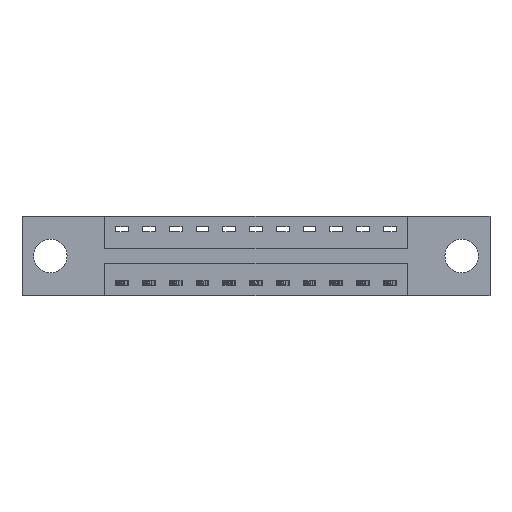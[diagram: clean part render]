
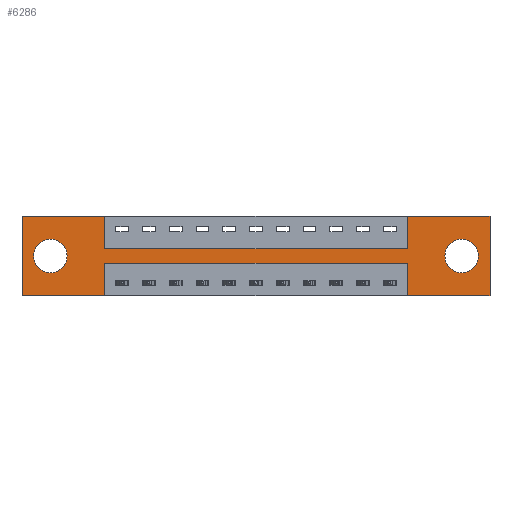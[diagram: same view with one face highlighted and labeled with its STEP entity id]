
A CAD part, front view. The second image highlights one B-rep face of the part: STEP entity #6286.
In plain terms, the highlighted planar face has unit normal (0, -1, 0).
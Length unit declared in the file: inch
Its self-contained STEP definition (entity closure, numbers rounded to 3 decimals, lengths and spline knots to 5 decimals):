
#177 = VERTEX_POINT ( 'NONE', #10046 ) ;
#226 = LINE ( 'NONE', #3728, #1477 ) ;
#584 = CARTESIAN_POINT ( 'NONE',  ( 2.0525, 0., -0.107 ) ) ;
#644 = DIRECTION ( 'NONE',  ( 1., 0., 0. ) ) ;
#660 = ORIENTED_EDGE ( 'NONE', *, *, #10519, .F. ) ;
#899 = DIRECTION ( 'NONE',  ( 0., 0., -1. ) ) ;
#930 = AXIS2_PLACEMENT_3D ( 'NONE', #1016, #8815, #899 ) ;
#969 = VERTEX_POINT ( 'NONE', #1313 ) ;
#1016 = CARTESIAN_POINT ( 'NONE',  ( 0., 0., -0.37 ) ) ;
#1032 = VERTEX_POINT ( 'NONE', #584 ) ;
#1133 = CARTESIAN_POINT ( 'NONE',  ( 0.3875, 0., -0.37 ) ) ;
#1294 = VECTOR ( 'NONE', #8413, 39.37008 ) ;
#1313 = CARTESIAN_POINT ( 'NONE',  ( 1.7975, 0., 0. ) ) ;
#1326 = VERTEX_POINT ( 'NONE', #6368 ) ;
#1356 = AXIS2_PLACEMENT_3D ( 'NONE', #8664, #11412, #7857 ) ;
#1359 = LINE ( 'NONE', #4847, #7010 ) ;
#1381 = VERTEX_POINT ( 'NONE', #1632 ) ;
#1389 = ORIENTED_EDGE ( 'NONE', *, *, #9630, .F. ) ;
#1477 = VECTOR ( 'NONE', #7262, 39.37008 ) ;
#1508 = DIRECTION ( 'NONE',  ( 1., 0., 0. ) ) ;
#1519 = VERTEX_POINT ( 'NONE', #1788 ) ;
#1606 = LINE ( 'NONE', #5100, #11289 ) ;
#1612 = AXIS2_PLACEMENT_3D ( 'NONE', #1941, #1887, #5586 ) ;
#1632 = CARTESIAN_POINT ( 'NONE',  ( 0.3875, 0., -0.37 ) ) ;
#1730 = LINE ( 'NONE', #2696, #7030 ) ;
#1788 = CARTESIAN_POINT ( 'NONE',  ( 0., 0., 0. ) ) ;
#1887 = DIRECTION ( 'NONE',  ( 0., 1., 0. ) ) ;
#1920 = CARTESIAN_POINT ( 'NONE',  ( 0., 0., -0.37 ) ) ;
#1927 = ORIENTED_EDGE ( 'NONE', *, *, #9929, .F. ) ;
#1941 = CARTESIAN_POINT ( 'NONE',  ( 2.0525, 0., -0.185 ) ) ;
#1965 = ORIENTED_EDGE ( 'NONE', *, *, #5904, .T. ) ;
#2039 = CARTESIAN_POINT ( 'NONE',  ( 2.0525, 0., -0.263 ) ) ;
#2087 = CARTESIAN_POINT ( 'NONE',  ( 0.1325, 0., -0.107 ) ) ;
#2130 = EDGE_CURVE ( 'NONE', #1032, #3331, #2693, .T. ) ;
#2263 = CARTESIAN_POINT ( 'NONE',  ( 2.185, 0., 0. ) ) ;
#2311 = DIRECTION ( 'NONE',  ( 0., 0., -1. ) ) ;
#2410 = VERTEX_POINT ( 'NONE', #5102 ) ;
#2524 = ORIENTED_EDGE ( 'NONE', *, *, #10858, .F. ) ;
#2571 = CIRCLE ( 'NONE', #7759, 0.078 ) ;
#2693 = CIRCLE ( 'NONE', #1612, 0.078 ) ;
#2696 = CARTESIAN_POINT ( 'NONE',  ( 0., 0., 0. ) ) ;
#2708 = FACE_BOUND ( 'NONE', #5541, .T. ) ;
#2937 = ORIENTED_EDGE ( 'NONE', *, *, #5645, .T. ) ;
#2990 = CIRCLE ( 'NONE', #9469, 0.078 ) ;
#2996 = CIRCLE ( 'NONE', #1356, 0.078 ) ;
#3052 = DIRECTION ( 'NONE',  ( -1., 0., 0. ) ) ;
#3071 = LINE ( 'NONE', #10981, #1294 ) ;
#3082 = VERTEX_POINT ( 'NONE', #5969 ) ;
#3173 = VECTOR ( 'NONE', #6557, 39.37008 ) ;
#3221 = CARTESIAN_POINT ( 'NONE',  ( 0.3875, 0., 0. ) ) ;
#3242 = ORIENTED_EDGE ( 'NONE', *, *, #7009, .F. ) ;
#3331 = VERTEX_POINT ( 'NONE', #2039 ) ;
#3390 = DIRECTION ( 'NONE',  ( -1., 0., 0. ) ) ;
#3644 = CARTESIAN_POINT ( 'NONE',  ( 1.7975, 0., 0. ) ) ;
#3651 = VERTEX_POINT ( 'NONE', #10027 ) ;
#3728 = CARTESIAN_POINT ( 'NONE',  ( 0.3875, 0., -0.15 ) ) ;
#3993 = ORIENTED_EDGE ( 'NONE', *, *, #8952, .F. ) ;
#4127 = EDGE_CURVE ( 'NONE', #3331, #1032, #2571, .T. ) ;
#4445 = DIRECTION ( 'NONE',  ( 0., 0., 1. ) ) ;
#4514 = EDGE_CURVE ( 'NONE', #1326, #177, #226, .T. ) ;
#4521 = DIRECTION ( 'NONE',  ( 0., 1., 0. ) ) ;
#4752 = CARTESIAN_POINT ( 'NONE',  ( 2.185, 0., 0. ) ) ;
#4847 = CARTESIAN_POINT ( 'NONE',  ( 1.7975, 0., -0.37 ) ) ;
#4942 = ORIENTED_EDGE ( 'NONE', *, *, #10510, .F. ) ;
#5100 = CARTESIAN_POINT ( 'NONE',  ( 0.3875, 0., -0.22 ) ) ;
#5102 = CARTESIAN_POINT ( 'NONE',  ( 0.3875, 0., -0.22 ) ) ;
#5174 = VERTEX_POINT ( 'NONE', #2263 ) ;
#5384 = CARTESIAN_POINT ( 'NONE',  ( 0.1325, 0., -0.185 ) ) ;
#5439 = DIRECTION ( 'NONE',  ( 0., 0., 1. ) ) ;
#5509 = CARTESIAN_POINT ( 'NONE',  ( 1.7975, 0., -0.22 ) ) ;
#5541 = EDGE_LOOP ( 'NONE', ( #9595, #7625 ) ) ;
#5564 = VECTOR ( 'NONE', #644, 39.37008 ) ;
#5586 = DIRECTION ( 'NONE',  ( 0., 0., -1. ) ) ;
#5645 = EDGE_CURVE ( 'NONE', #3651, #9729, #2996, .T. ) ;
#5826 = ORIENTED_EDGE ( 'NONE', *, *, #11350, .F. ) ;
#5897 = VERTEX_POINT ( 'NONE', #1920 ) ;
#5904 = EDGE_CURVE ( 'NONE', #9729, #3651, #2990, .T. ) ;
#5969 = CARTESIAN_POINT ( 'NONE',  ( 0.3875, 0., 0. ) ) ;
#6031 = ORIENTED_EDGE ( 'NONE', *, *, #8406, .F. ) ;
#6286 = ADVANCED_FACE ( 'NONE', ( #2708, #9049, #8123 ), #8930, .T. ) ;
#6368 = CARTESIAN_POINT ( 'NONE',  ( 0.3875, 0., -0.15 ) ) ;
#6425 = DIRECTION ( 'NONE',  ( 0., 0., 1. ) ) ;
#6510 = CARTESIAN_POINT ( 'NONE',  ( 2.0525, 0., -0.185 ) ) ;
#6557 = DIRECTION ( 'NONE',  ( 0., 0., -1. ) ) ;
#6595 = EDGE_CURVE ( 'NONE', #5897, #1519, #1730, .T. ) ;
#6652 = VECTOR ( 'NONE', #10560, 39.37008 ) ;
#6675 = CARTESIAN_POINT ( 'NONE',  ( 0., 0., 0. ) ) ;
#6992 = ORIENTED_EDGE ( 'NONE', *, *, #6595, .F. ) ;
#7003 = EDGE_LOOP ( 'NONE', ( #1965, #2937 ) ) ;
#7009 = EDGE_CURVE ( 'NONE', #969, #5174, #10257, .T. ) ;
#7010 = VECTOR ( 'NONE', #6425, 39.37008 ) ;
#7030 = VECTOR ( 'NONE', #4445, 39.37008 ) ;
#7059 = EDGE_CURVE ( 'NONE', #3082, #1326, #11187, .T. ) ;
#7063 = LINE ( 'NONE', #3644, #6652 ) ;
#7262 = DIRECTION ( 'NONE',  ( 1., 0., 0. ) ) ;
#7466 = LINE ( 'NONE', #11018, #9976 ) ;
#7625 = ORIENTED_EDGE ( 'NONE', *, *, #4127, .T. ) ;
#7674 = LINE ( 'NONE', #4752, #3173 ) ;
#7759 = AXIS2_PLACEMENT_3D ( 'NONE', #6510, #10012, #9296 ) ;
#7857 = DIRECTION ( 'NONE',  ( 0., 0., 1. ) ) ;
#8123 = FACE_OUTER_BOUND ( 'NONE', #10546, .T. ) ;
#8166 = VECTOR ( 'NONE', #10314, 39.37008 ) ;
#8311 = VERTEX_POINT ( 'NONE', #8400 ) ;
#8400 = CARTESIAN_POINT ( 'NONE',  ( 2.185, 0., -0.37 ) ) ;
#8406 = EDGE_CURVE ( 'NONE', #2410, #1381, #10142, .T. ) ;
#8413 = DIRECTION ( 'NONE',  ( -1., 0., 0. ) ) ;
#8664 = CARTESIAN_POINT ( 'NONE',  ( 0.1325, 0., -0.185 ) ) ;
#8815 = DIRECTION ( 'NONE',  ( 0., -1., 0. ) ) ;
#8930 = PLANE ( 'NONE',  #930 ) ;
#8952 = EDGE_CURVE ( 'NONE', #9031, #2410, #1606, .T. ) ;
#9031 = VERTEX_POINT ( 'NONE', #5509 ) ;
#9049 = FACE_BOUND ( 'NONE', #7003, .T. ) ;
#9196 = ORIENTED_EDGE ( 'NONE', *, *, #4514, .F. ) ;
#9256 = CARTESIAN_POINT ( 'NONE',  ( 0., 0., 0. ) ) ;
#9296 = DIRECTION ( 'NONE',  ( 0., 0., -1. ) ) ;
#9469 = AXIS2_PLACEMENT_3D ( 'NONE', #5384, #4521, #5439 ) ;
#9595 = ORIENTED_EDGE ( 'NONE', *, *, #2130, .T. ) ;
#9630 = EDGE_CURVE ( 'NONE', #11240, #9031, #1359, .T. ) ;
#9729 = VERTEX_POINT ( 'NONE', #2087 ) ;
#9929 = EDGE_CURVE ( 'NONE', #177, #969, #7063, .T. ) ;
#9976 = VECTOR ( 'NONE', #3052, 39.37008 ) ;
#10012 = DIRECTION ( 'NONE',  ( 0., 1., 0. ) ) ;
#10027 = CARTESIAN_POINT ( 'NONE',  ( 0.1325, 0., -0.263 ) ) ;
#10033 = CARTESIAN_POINT ( 'NONE',  ( 1.7975, 0., -0.37 ) ) ;
#10046 = CARTESIAN_POINT ( 'NONE',  ( 1.7975, 0., -0.15 ) ) ;
#10118 = VECTOR ( 'NONE', #2311, 39.37008 ) ;
#10142 = LINE ( 'NONE', #1133, #10118 ) ;
#10257 = LINE ( 'NONE', #9256, #10570 ) ;
#10314 = DIRECTION ( 'NONE',  ( 0., 0., -1. ) ) ;
#10510 = EDGE_CURVE ( 'NONE', #5174, #8311, #7674, .T. ) ;
#10519 = EDGE_CURVE ( 'NONE', #1519, #3082, #11054, .T. ) ;
#10546 = EDGE_LOOP ( 'NONE', ( #6031, #3993, #1389, #5826, #4942, #3242, #1927, #9196, #11329, #660, #6992, #2524 ) ) ;
#10560 = DIRECTION ( 'NONE',  ( 0., 0., 1. ) ) ;
#10570 = VECTOR ( 'NONE', #1508, 39.37008 ) ;
#10858 = EDGE_CURVE ( 'NONE', #1381, #5897, #3071, .T. ) ;
#10981 = CARTESIAN_POINT ( 'NONE',  ( 0., 0., -0.37 ) ) ;
#11018 = CARTESIAN_POINT ( 'NONE',  ( 0., 0., -0.37 ) ) ;
#11054 = LINE ( 'NONE', #6675, #5564 ) ;
#11187 = LINE ( 'NONE', #3221, #8166 ) ;
#11240 = VERTEX_POINT ( 'NONE', #10033 ) ;
#11289 = VECTOR ( 'NONE', #3390, 39.37008 ) ;
#11329 = ORIENTED_EDGE ( 'NONE', *, *, #7059, .F. ) ;
#11350 = EDGE_CURVE ( 'NONE', #8311, #11240, #7466, .T. ) ;
#11412 = DIRECTION ( 'NONE',  ( 0., 1., 0. ) ) ;
